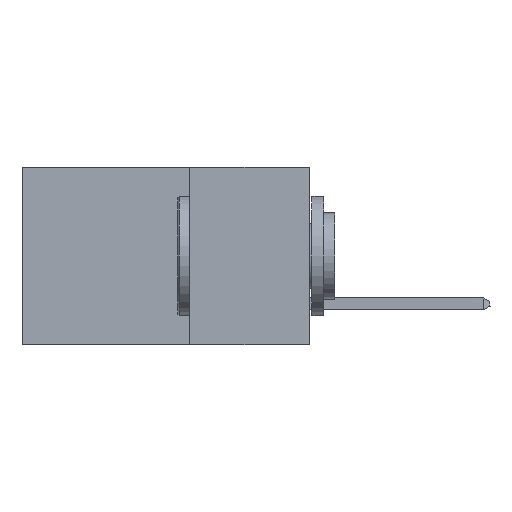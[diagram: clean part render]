
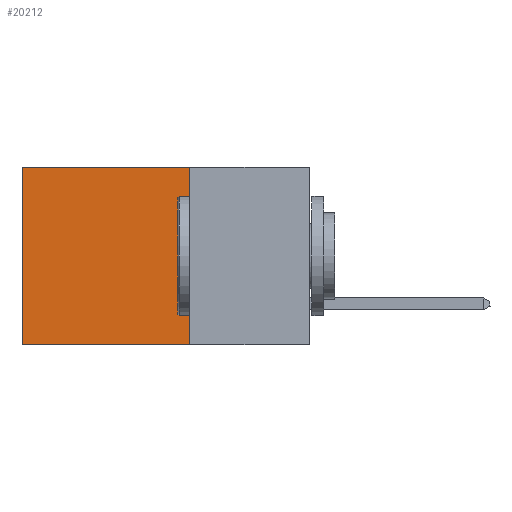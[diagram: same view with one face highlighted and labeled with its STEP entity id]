
A CAD part, left-side view. The second image highlights one B-rep face of the part: STEP entity #20212.
In plain terms, the highlighted planar face has unit normal (-1, 0, 0).
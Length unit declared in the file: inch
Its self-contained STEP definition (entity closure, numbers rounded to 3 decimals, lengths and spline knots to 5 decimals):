
#1594 = DIRECTION ( 'NONE',  ( 0., 1., 0. ) ) ;
#2606 = ORIENTED_EDGE ( 'NONE', *, *, #18632, .T. ) ;
#4105 = ORIENTED_EDGE ( 'NONE', *, *, #25819, .F. ) ;
#6025 = LINE ( 'NONE', #25300, #16554 ) ;
#6160 = LINE ( 'NONE', #21070, #27649 ) ;
#6315 = DIRECTION ( 'NONE',  ( 0., 0., -1. ) ) ;
#7099 = LINE ( 'NONE', #8528, #7486 ) ;
#7486 = VECTOR ( 'NONE', #28012, 39.37008 ) ;
#8528 = CARTESIAN_POINT ( 'NONE',  ( 0.2875, 0.25, -0.37 ) ) ;
#9662 = DIRECTION ( 'NONE',  ( 0., 0., -1. ) ) ;
#9862 = CARTESIAN_POINT ( 'NONE',  ( 0.2875, 0.25, -0.37 ) ) ;
#9914 = VERTEX_POINT ( 'NONE', #23341 ) ;
#10011 = VERTEX_POINT ( 'NONE', #12963 ) ;
#10886 = EDGE_CURVE ( 'NONE', #27633, #9914, #6025, .T. ) ;
#11120 = FACE_OUTER_BOUND ( 'NONE', #31945, .T. ) ;
#11805 = CARTESIAN_POINT ( 'NONE',  ( 0.2875, 0.25, 0. ) ) ;
#12720 = VECTOR ( 'NONE', #6315, 39.37008 ) ;
#12963 = CARTESIAN_POINT ( 'NONE',  ( 0.2875, 0.6, -0.37 ) ) ;
#14332 = PLANE ( 'NONE',  #23555 ) ;
#14794 = ORIENTED_EDGE ( 'NONE', *, *, #10886, .T. ) ;
#15586 = DIRECTION ( 'NONE',  ( 0., 0., -1. ) ) ;
#16554 = VECTOR ( 'NONE', #1594, 39.37008 ) ;
#18632 = EDGE_CURVE ( 'NONE', #9914, #10011, #6160, .T. ) ;
#20212 = ADVANCED_FACE ( 'NONE', ( #11120 ), #14332, .F. ) ;
#20268 = VERTEX_POINT ( 'NONE', #9862 ) ;
#21070 = CARTESIAN_POINT ( 'NONE',  ( 0.2875, 0.6, 0. ) ) ;
#21291 = CARTESIAN_POINT ( 'NONE',  ( 0.2875, 0.25, 0. ) ) ;
#21390 = LINE ( 'NONE', #21291, #12720 ) ;
#23341 = CARTESIAN_POINT ( 'NONE',  ( 0.2875, 0.6, 0. ) ) ;
#23555 = AXIS2_PLACEMENT_3D ( 'NONE', #11805, #24569, #9662 ) ;
#24569 = DIRECTION ( 'NONE',  ( 1., 0., 0. ) ) ;
#25300 = CARTESIAN_POINT ( 'NONE',  ( 0.2875, 0.25, 0. ) ) ;
#25819 = EDGE_CURVE ( 'NONE', #27633, #20268, #21390, .T. ) ;
#26263 = ORIENTED_EDGE ( 'NONE', *, *, #28560, .F. ) ;
#27633 = VERTEX_POINT ( 'NONE', #28250 ) ;
#27649 = VECTOR ( 'NONE', #15586, 39.37008 ) ;
#28012 = DIRECTION ( 'NONE',  ( 0., 1., 0. ) ) ;
#28250 = CARTESIAN_POINT ( 'NONE',  ( 0.2875, 0.25, 0. ) ) ;
#28560 = EDGE_CURVE ( 'NONE', #20268, #10011, #7099, .T. ) ;
#31945 = EDGE_LOOP ( 'NONE', ( #2606, #26263, #4105, #14794 ) ) ;
